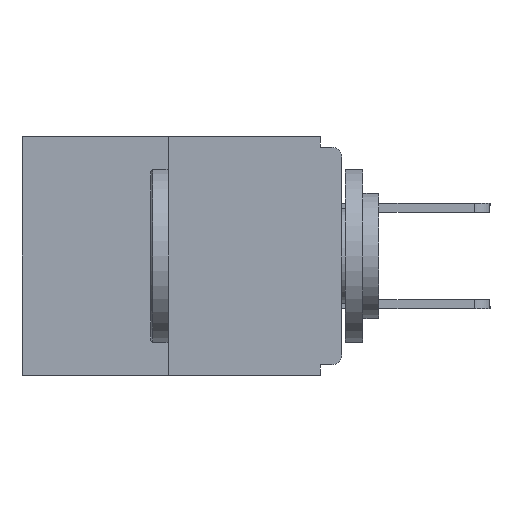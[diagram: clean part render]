
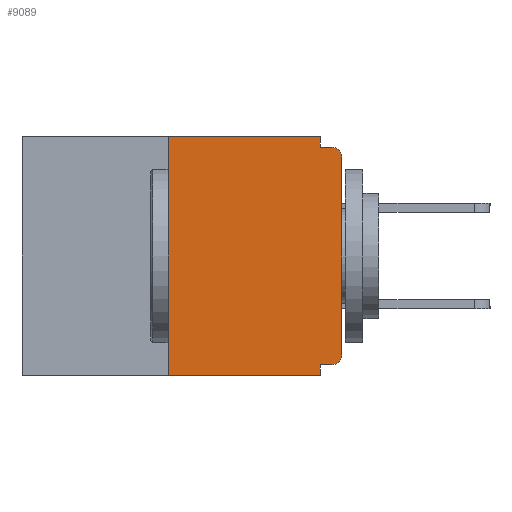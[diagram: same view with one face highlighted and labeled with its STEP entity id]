
A CAD part, left-side view. The second image highlights one B-rep face of the part: STEP entity #9089.
In plain terms, the highlighted planar face has unit normal (-1, 0, 0).
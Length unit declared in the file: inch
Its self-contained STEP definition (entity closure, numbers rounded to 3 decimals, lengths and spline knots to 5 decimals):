
#372 = VECTOR ( 'NONE', #2305, 39.37008 ) ;
#643 = VECTOR ( 'NONE', #11611, 39.37008 ) ;
#726 = CARTESIAN_POINT ( 'NONE',  ( 0., 0.25, 0. ) ) ;
#1053 = DIRECTION ( 'NONE',  ( 0., -1., 0. ) ) ;
#1244 = VERTEX_POINT ( 'NONE', #24878 ) ;
#1889 = PLANE ( 'NONE',  #25036 ) ;
#2096 = CARTESIAN_POINT ( 'NONE',  ( 0., 0.015, -0.313 ) ) ;
#2272 = ORIENTED_EDGE ( 'NONE', *, *, #4957, .F. ) ;
#2305 = DIRECTION ( 'NONE',  ( 0., -1., 0. ) ) ;
#2567 = CARTESIAN_POINT ( 'NONE',  ( 0., 0.031, -0.015 ) ) ;
#2600 = LINE ( 'NONE', #7208, #22724 ) ;
#3729 = CARTESIAN_POINT ( 'NONE',  ( 0., 0.031, 0. ) ) ;
#3759 = LINE ( 'NONE', #4040, #10180 ) ;
#3817 = DIRECTION ( 'NONE',  ( 0., 0., -1. ) ) ;
#4040 = CARTESIAN_POINT ( 'NONE',  ( 0., 0.46, 0. ) ) ;
#4957 = EDGE_CURVE ( 'NONE', #18531, #18944, #6641, .T. ) ;
#5667 = EDGE_CURVE ( 'NONE', #24232, #20162, #23800, .T. ) ;
#6142 = DIRECTION ( 'NONE',  ( 0., -1., 0. ) ) ;
#6530 = EDGE_CURVE ( 'NONE', #9772, #14096, #9080, .T. ) ;
#6641 = LINE ( 'NONE', #12789, #21372 ) ;
#7162 = EDGE_CURVE ( 'NONE', #9772, #18944, #11538, .T. ) ;
#7208 = CARTESIAN_POINT ( 'NONE',  ( 0., 0., 0. ) ) ;
#7390 = CARTESIAN_POINT ( 'NONE',  ( 0., 0., -0.03 ) ) ;
#7485 = ORIENTED_EDGE ( 'NONE', *, *, #7162, .T. ) ;
#7985 = ORIENTED_EDGE ( 'NONE', *, *, #6530, .F. ) ;
#8949 = ORIENTED_EDGE ( 'NONE', *, *, #5667, .T. ) ;
#9080 = LINE ( 'NONE', #19964, #19181 ) ;
#9089 = ADVANCED_FACE ( 'NONE', ( #22391 ), #1889, .F. ) ;
#9330 = ORIENTED_EDGE ( 'NONE', *, *, #22371, .F. ) ;
#9391 = CARTESIAN_POINT ( 'NONE',  ( 0., 0.015, -0.03 ) ) ;
#9661 = CARTESIAN_POINT ( 'NONE',  ( 0., 0.031, -0.328 ) ) ;
#9772 = VERTEX_POINT ( 'NONE', #20799 ) ;
#9964 = EDGE_CURVE ( 'NONE', #19644, #20162, #16837, .T. ) ;
#10180 = VECTOR ( 'NONE', #6142, 39.37008 ) ;
#10200 = VERTEX_POINT ( 'NONE', #14300 ) ;
#10532 = ORIENTED_EDGE ( 'NONE', *, *, #12438, .T. ) ;
#10572 = DIRECTION ( 'NONE',  ( 0., 0., -1. ) ) ;
#10694 = VERTEX_POINT ( 'NONE', #19584 ) ;
#11347 = DIRECTION ( 'NONE',  ( 0., 0., 1. ) ) ;
#11538 = LINE ( 'NONE', #24448, #22813 ) ;
#11611 = DIRECTION ( 'NONE',  ( 0., 0., -1. ) ) ;
#12438 = EDGE_CURVE ( 'NONE', #10694, #1244, #18168, .T. ) ;
#12545 = CARTESIAN_POINT ( 'NONE',  ( 0., 0.015, -0.015 ) ) ;
#12789 = CARTESIAN_POINT ( 'NONE',  ( 0., 0.031, -0.343 ) ) ;
#13521 = EDGE_LOOP ( 'NONE', ( #22399, #7985, #7485, #2272, #9330, #10532, #21779, #8949, #15200, #13856 ) ) ;
#13851 = DIRECTION ( 'NONE',  ( 0., 0., -1. ) ) ;
#13856 = ORIENTED_EDGE ( 'NONE', *, *, #23222, .F. ) ;
#14031 = DIRECTION ( 'NONE',  ( -1., 0., 0. ) ) ;
#14096 = VERTEX_POINT ( 'NONE', #726 ) ;
#14300 = CARTESIAN_POINT ( 'NONE',  ( 0., 0.031, 0. ) ) ;
#14740 = DIRECTION ( 'NONE',  ( 0., 1., 0. ) ) ;
#15200 = ORIENTED_EDGE ( 'NONE', *, *, #9964, .F. ) ;
#16141 = DIRECTION ( 'NONE',  ( 0., 0., 1. ) ) ;
#16837 = LINE ( 'NONE', #20033, #372 ) ;
#18168 = CIRCLE ( 'NONE', #23689, 0.015 ) ;
#18531 = VERTEX_POINT ( 'NONE', #9661 ) ;
#18944 = VERTEX_POINT ( 'NONE', #22000 ) ;
#19181 = VECTOR ( 'NONE', #16141, 39.37008 ) ;
#19584 = CARTESIAN_POINT ( 'NONE',  ( 0., 0.015, -0.328 ) ) ;
#19644 = VERTEX_POINT ( 'NONE', #2567 ) ;
#19964 = CARTESIAN_POINT ( 'NONE',  ( 0., 0.25, 0. ) ) ;
#20033 = CARTESIAN_POINT ( 'NONE',  ( 0., 0., -0.015 ) ) ;
#20162 = VERTEX_POINT ( 'NONE', #12545 ) ;
#20334 = EDGE_CURVE ( 'NONE', #1244, #24232, #2600, .T. ) ;
#20799 = CARTESIAN_POINT ( 'NONE',  ( 0., 0.25, -0.343 ) ) ;
#21246 = CARTESIAN_POINT ( 'NONE',  ( 0., 0.46, 0. ) ) ;
#21372 = VECTOR ( 'NONE', #10572, 39.37008 ) ;
#21431 = LINE ( 'NONE', #3729, #643 ) ;
#21779 = ORIENTED_EDGE ( 'NONE', *, *, #20334, .T. ) ;
#22000 = CARTESIAN_POINT ( 'NONE',  ( 0., 0.031, -0.343 ) ) ;
#22371 = EDGE_CURVE ( 'NONE', #10694, #18531, #23009, .T. ) ;
#22391 = FACE_OUTER_BOUND ( 'NONE', #13521, .T. ) ;
#22399 = ORIENTED_EDGE ( 'NONE', *, *, #25183, .F. ) ;
#22688 = CARTESIAN_POINT ( 'NONE',  ( 0., 0., -0.328 ) ) ;
#22724 = VECTOR ( 'NONE', #11347, 39.37008 ) ;
#22802 = DIRECTION ( 'NONE',  ( -1., 0., 0. ) ) ;
#22813 = VECTOR ( 'NONE', #1053, 39.37008 ) ;
#23009 = LINE ( 'NONE', #22688, #25121 ) ;
#23222 = EDGE_CURVE ( 'NONE', #10200, #19644, #21431, .T. ) ;
#23234 = AXIS2_PLACEMENT_3D ( 'NONE', #9391, #22802, #24676 ) ;
#23689 = AXIS2_PLACEMENT_3D ( 'NONE', #2096, #14031, #13851 ) ;
#23800 = CIRCLE ( 'NONE', #23234, 0.015 ) ;
#24232 = VERTEX_POINT ( 'NONE', #7390 ) ;
#24448 = CARTESIAN_POINT ( 'NONE',  ( 0., 0.46, -0.343 ) ) ;
#24676 = DIRECTION ( 'NONE',  ( 0., 0., -1. ) ) ;
#24878 = CARTESIAN_POINT ( 'NONE',  ( 0., 0., -0.313 ) ) ;
#25036 = AXIS2_PLACEMENT_3D ( 'NONE', #21246, #25171, #3817 ) ;
#25121 = VECTOR ( 'NONE', #14740, 39.37008 ) ;
#25171 = DIRECTION ( 'NONE',  ( 1., 0., 0. ) ) ;
#25183 = EDGE_CURVE ( 'NONE', #14096, #10200, #3759, .T. ) ;
